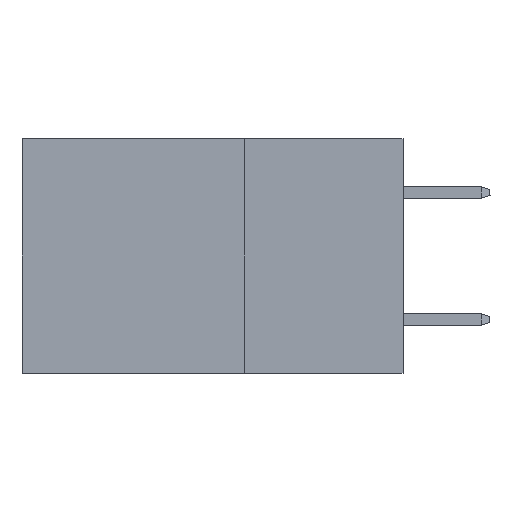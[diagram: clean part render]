
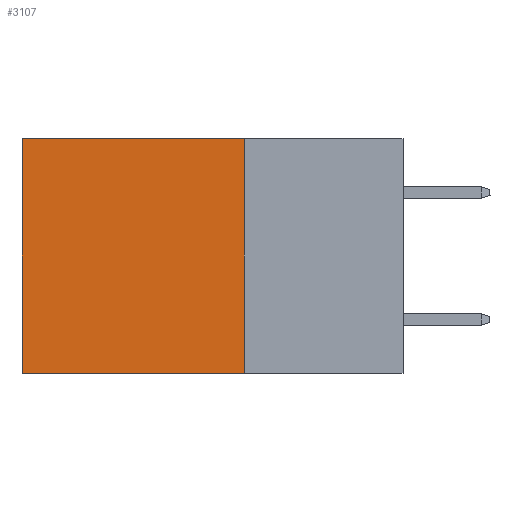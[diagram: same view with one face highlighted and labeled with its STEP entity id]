
A CAD part, left-side view. The second image highlights one B-rep face of the part: STEP entity #3107.
In plain terms, the highlighted planar face has unit normal (-1, 0, 0).
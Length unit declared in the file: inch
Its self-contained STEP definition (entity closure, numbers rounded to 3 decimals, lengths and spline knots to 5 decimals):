
#656 = PLANE ( 'NONE',  #34596 ) ;
#737 = CARTESIAN_POINT ( 'NONE',  ( 0.2875, 0.25, 0. ) ) ;
#795 = VECTOR ( 'NONE', #5576, 39.37008 ) ;
#845 = VECTOR ( 'NONE', #34299, 39.37008 ) ;
#1952 = CARTESIAN_POINT ( 'NONE',  ( 0.2875, 0.6, -0.37 ) ) ;
#2754 = ORIENTED_EDGE ( 'NONE', *, *, #12423, .F. ) ;
#3107 = ADVANCED_FACE ( 'NONE', ( #5890 ), #656, .F. ) ;
#3297 = VERTEX_POINT ( 'NONE', #34207 ) ;
#3725 = CARTESIAN_POINT ( 'NONE',  ( 0.2875, 0.25, -0.37 ) ) ;
#4663 = ORIENTED_EDGE ( 'NONE', *, *, #13488, .T. ) ;
#5576 = DIRECTION ( 'NONE',  ( 0., 1., 0. ) ) ;
#5890 = FACE_OUTER_BOUND ( 'NONE', #33516, .T. ) ;
#6326 = DIRECTION ( 'NONE',  ( 0., 0., -1. ) ) ;
#6971 = LINE ( 'NONE', #17962, #23036 ) ;
#9312 = DIRECTION ( 'NONE',  ( 1., 0., 0. ) ) ;
#10995 = LINE ( 'NONE', #16733, #795 ) ;
#11202 = VERTEX_POINT ( 'NONE', #3725 ) ;
#12423 = EDGE_CURVE ( 'NONE', #11202, #26220, #10995, .T. ) ;
#13284 = VECTOR ( 'NONE', #6326, 39.37008 ) ;
#13488 = EDGE_CURVE ( 'NONE', #3297, #14761, #31424, .T. ) ;
#14761 = VERTEX_POINT ( 'NONE', #25508 ) ;
#15604 = ORIENTED_EDGE ( 'NONE', *, *, #20889, .T. ) ;
#16733 = CARTESIAN_POINT ( 'NONE',  ( 0.2875, 0.25, -0.37 ) ) ;
#16953 = LINE ( 'NONE', #737, #13284 ) ;
#17227 = CARTESIAN_POINT ( 'NONE',  ( 0.2875, 0.25, 0. ) ) ;
#17676 = CARTESIAN_POINT ( 'NONE',  ( 0.2875, 0.25, 0. ) ) ;
#17962 = CARTESIAN_POINT ( 'NONE',  ( 0.2875, 0.6, 0. ) ) ;
#20889 = EDGE_CURVE ( 'NONE', #14761, #26220, #6971, .T. ) ;
#23036 = VECTOR ( 'NONE', #29016, 39.37008 ) ;
#25508 = CARTESIAN_POINT ( 'NONE',  ( 0.2875, 0.6, 0. ) ) ;
#26220 = VERTEX_POINT ( 'NONE', #1952 ) ;
#28294 = DIRECTION ( 'NONE',  ( 0., 0., -1. ) ) ;
#28666 = EDGE_CURVE ( 'NONE', #3297, #11202, #16953, .T. ) ;
#29016 = DIRECTION ( 'NONE',  ( 0., 0., -1. ) ) ;
#29710 = ORIENTED_EDGE ( 'NONE', *, *, #28666, .F. ) ;
#31424 = LINE ( 'NONE', #17676, #845 ) ;
#33516 = EDGE_LOOP ( 'NONE', ( #15604, #2754, #29710, #4663 ) ) ;
#34207 = CARTESIAN_POINT ( 'NONE',  ( 0.2875, 0.25, 0. ) ) ;
#34299 = DIRECTION ( 'NONE',  ( 0., 1., 0. ) ) ;
#34596 = AXIS2_PLACEMENT_3D ( 'NONE', #17227, #9312, #28294 ) ;
